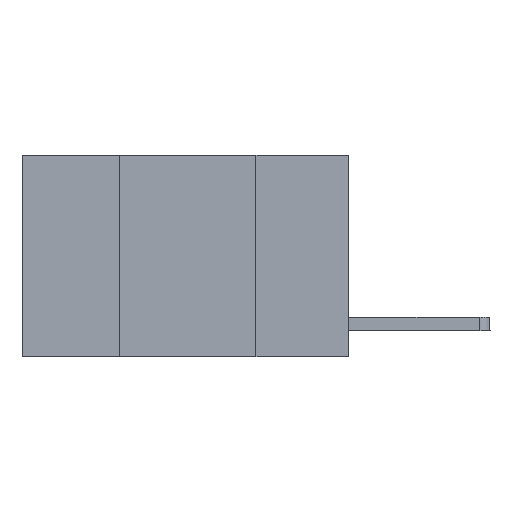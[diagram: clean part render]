
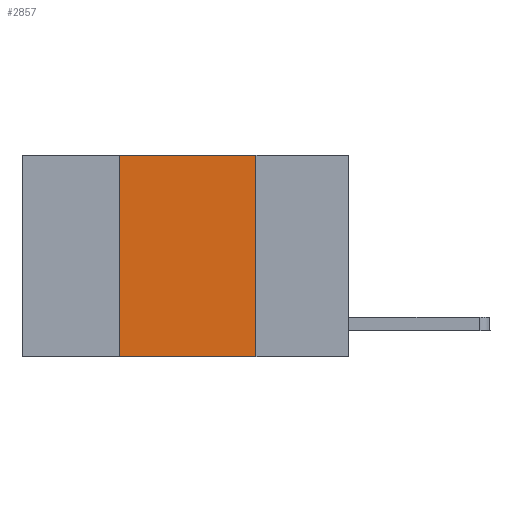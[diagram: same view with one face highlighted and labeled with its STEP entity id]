
A CAD part, left-side view. The second image highlights one B-rep face of the part: STEP entity #2857.
In plain terms, the highlighted planar face has unit normal (-1, 0, 0).
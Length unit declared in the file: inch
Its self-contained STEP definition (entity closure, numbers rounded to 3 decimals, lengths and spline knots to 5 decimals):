
#277 = CARTESIAN_POINT ( 'NONE',  ( 0., 0.6, 0. ) ) ;
#498 = DIRECTION ( 'NONE',  ( 0., -1., 0. ) ) ;
#595 = VERTEX_POINT ( 'NONE', #2864 ) ;
#662 = EDGE_LOOP ( 'NONE', ( #4268, #6071, #5923, #1624 ) ) ;
#1032 = CARTESIAN_POINT ( 'NONE',  ( 0., 0.17, 0. ) ) ;
#1271 = CARTESIAN_POINT ( 'NONE',  ( 0., 0.17, -0.37 ) ) ;
#1624 = ORIENTED_EDGE ( 'NONE', *, *, #8717, .T. ) ;
#1719 = VECTOR ( 'NONE', #498, 39.37008 ) ;
#1722 = VECTOR ( 'NONE', #3854, 39.37008 ) ;
#2052 = DIRECTION ( 'NONE',  ( 0., 0., -1. ) ) ;
#2450 = CARTESIAN_POINT ( 'NONE',  ( 0., 0.42, 0. ) ) ;
#2680 = CARTESIAN_POINT ( 'NONE',  ( 0., 0.17, 0. ) ) ;
#2857 = ADVANCED_FACE ( 'NONE', ( #6121 ), #4815, .F. ) ;
#2864 = CARTESIAN_POINT ( 'NONE',  ( 0., 0.42, 0. ) ) ;
#3122 = VERTEX_POINT ( 'NONE', #7387 ) ;
#3283 = VECTOR ( 'NONE', #5651, 39.37008 ) ;
#3365 = LINE ( 'NONE', #2680, #3283 ) ;
#3591 = AXIS2_PLACEMENT_3D ( 'NONE', #6847, #8928, #2052 ) ;
#3854 = DIRECTION ( 'NONE',  ( 0., -1., 0. ) ) ;
#3939 = CARTESIAN_POINT ( 'NONE',  ( 0., 0.6, -0.37 ) ) ;
#4092 = VECTOR ( 'NONE', #6559, 39.37008 ) ;
#4268 = ORIENTED_EDGE ( 'NONE', *, *, #5407, .F. ) ;
#4428 = LINE ( 'NONE', #2450, #4092 ) ;
#4815 = PLANE ( 'NONE',  #3591 ) ;
#5407 = EDGE_CURVE ( 'NONE', #6806, #7577, #3365, .T. ) ;
#5651 = DIRECTION ( 'NONE',  ( 0., 0., -1. ) ) ;
#5923 = ORIENTED_EDGE ( 'NONE', *, *, #8081, .F. ) ;
#5947 = LINE ( 'NONE', #277, #1722 ) ;
#6001 = EDGE_CURVE ( 'NONE', #595, #6806, #5947, .T. ) ;
#6071 = ORIENTED_EDGE ( 'NONE', *, *, #6001, .F. ) ;
#6121 = FACE_OUTER_BOUND ( 'NONE', #662, .T. ) ;
#6559 = DIRECTION ( 'NONE',  ( 0., 0., 1. ) ) ;
#6806 = VERTEX_POINT ( 'NONE', #1032 ) ;
#6847 = CARTESIAN_POINT ( 'NONE',  ( 0., 0.6, 0. ) ) ;
#7387 = CARTESIAN_POINT ( 'NONE',  ( 0., 0.42, -0.37 ) ) ;
#7577 = VERTEX_POINT ( 'NONE', #1271 ) ;
#8081 = EDGE_CURVE ( 'NONE', #3122, #595, #4428, .T. ) ;
#8113 = LINE ( 'NONE', #3939, #1719 ) ;
#8717 = EDGE_CURVE ( 'NONE', #3122, #7577, #8113, .T. ) ;
#8928 = DIRECTION ( 'NONE',  ( 1., 0., 0. ) ) ;
